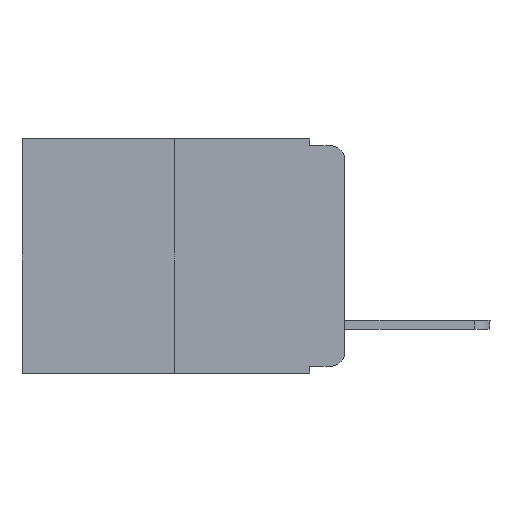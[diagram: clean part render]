
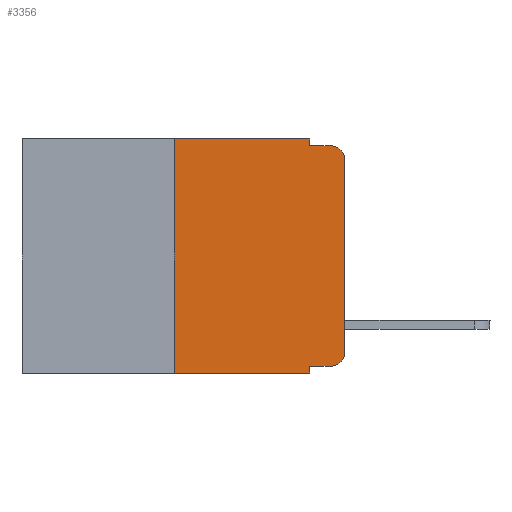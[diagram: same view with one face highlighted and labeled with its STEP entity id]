
A CAD part, left-side view. The second image highlights one B-rep face of the part: STEP entity #3356.
In plain terms, the highlighted planar face has unit normal (-1, 0, 0).
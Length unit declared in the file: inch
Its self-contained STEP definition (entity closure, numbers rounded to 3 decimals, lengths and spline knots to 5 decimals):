
#516 = CARTESIAN_POINT ( 'NONE',  ( 0., 0.051, 0. ) ) ;
#1097 = ORIENTED_EDGE ( 'NONE', *, *, #15260, .T. ) ;
#1399 = ORIENTED_EDGE ( 'NONE', *, *, #3674, .T. ) ;
#1534 = ORIENTED_EDGE ( 'NONE', *, *, #3552, .F. ) ;
#1713 = DIRECTION ( 'NONE',  ( -1., 0., 0. ) ) ;
#1716 = VERTEX_POINT ( 'NONE', #16718 ) ;
#1744 = LINE ( 'NONE', #8756, #10401 ) ;
#1872 = VECTOR ( 'NONE', #21773, 39.37008 ) ;
#2491 = PLANE ( 'NONE',  #20448 ) ;
#3356 = ADVANCED_FACE ( 'NONE', ( #13318 ), #2491, .F. ) ;
#3552 = EDGE_CURVE ( 'NONE', #8922, #5358, #19189, .T. ) ;
#3663 = DIRECTION ( 'NONE',  ( 0., 0., -1. ) ) ;
#3674 = EDGE_CURVE ( 'NONE', #6795, #16338, #4613, .T. ) ;
#3752 = CARTESIAN_POINT ( 'NONE',  ( 0., 0.473, -0.343 ) ) ;
#4172 = LINE ( 'NONE', #10744, #17664 ) ;
#4387 = DIRECTION ( 'NONE',  ( 0., 0., 1. ) ) ;
#4613 = LINE ( 'NONE', #11627, #20849 ) ;
#5263 = CARTESIAN_POINT ( 'NONE',  ( 0., 0.051, -0.333 ) ) ;
#5289 = CARTESIAN_POINT ( 'NONE',  ( 0., 0.02, -0.03 ) ) ;
#5358 = VERTEX_POINT ( 'NONE', #12371 ) ;
#5417 = CARTESIAN_POINT ( 'NONE',  ( 0., 0.25, -0.343 ) ) ;
#5496 = DIRECTION ( 'NONE',  ( 0., 0., -1. ) ) ;
#5788 = ORIENTED_EDGE ( 'NONE', *, *, #20070, .F. ) ;
#6242 = CARTESIAN_POINT ( 'NONE',  ( 0., 0.051, -0.01 ) ) ;
#6542 = VERTEX_POINT ( 'NONE', #11509 ) ;
#6795 = VERTEX_POINT ( 'NONE', #7782 ) ;
#7373 = ORIENTED_EDGE ( 'NONE', *, *, #12105, .T. ) ;
#7429 = DIRECTION ( 'NONE',  ( 0., -1., 0. ) ) ;
#7522 = DIRECTION ( 'NONE',  ( 0., 0., -1. ) ) ;
#7782 = CARTESIAN_POINT ( 'NONE',  ( 0., 0., -0.313 ) ) ;
#8155 = CIRCLE ( 'NONE', #21067, 0.02 ) ;
#8575 = ORIENTED_EDGE ( 'NONE', *, *, #13396, .F. ) ;
#8756 = CARTESIAN_POINT ( 'NONE',  ( 0., 0.473, 0. ) ) ;
#8760 = CARTESIAN_POINT ( 'NONE',  ( 0., 0.051, 0. ) ) ;
#8922 = VERTEX_POINT ( 'NONE', #6242 ) ;
#8944 = CARTESIAN_POINT ( 'NONE',  ( 0., 0.02, -0.313 ) ) ;
#8968 = VECTOR ( 'NONE', #5496, 39.37008 ) ;
#9504 = CARTESIAN_POINT ( 'NONE',  ( 0., 0.473, 0. ) ) ;
#9897 = CIRCLE ( 'NONE', #20600, 0.02 ) ;
#10401 = VECTOR ( 'NONE', #15806, 39.37008 ) ;
#10744 = CARTESIAN_POINT ( 'NONE',  ( 0., 0.051, 0. ) ) ;
#10857 = DIRECTION ( 'NONE',  ( 0., -1., 0. ) ) ;
#10921 = ORIENTED_EDGE ( 'NONE', *, *, #19192, .T. ) ;
#11509 = CARTESIAN_POINT ( 'NONE',  ( 0., 0.051, -0.333 ) ) ;
#11609 = CARTESIAN_POINT ( 'NONE',  ( 0., 0.25, 0. ) ) ;
#11627 = CARTESIAN_POINT ( 'NONE',  ( 0., 0., 0. ) ) ;
#11694 = VERTEX_POINT ( 'NONE', #5417 ) ;
#11960 = CARTESIAN_POINT ( 'NONE',  ( 0., 0.02, -0.333 ) ) ;
#12104 = CARTESIAN_POINT ( 'NONE',  ( 0., 0., -0.03 ) ) ;
#12105 = EDGE_CURVE ( 'NONE', #6542, #20189, #21035, .T. ) ;
#12227 = VECTOR ( 'NONE', #17567, 39.37008 ) ;
#12371 = CARTESIAN_POINT ( 'NONE',  ( 0., 0.02, -0.01 ) ) ;
#13111 = VECTOR ( 'NONE', #10857, 39.37008 ) ;
#13318 = FACE_OUTER_BOUND ( 'NONE', #18379, .T. ) ;
#13396 = EDGE_CURVE ( 'NONE', #6542, #19895, #21491, .T. ) ;
#14320 = ORIENTED_EDGE ( 'NONE', *, *, #17870, .F. ) ;
#14791 = ORIENTED_EDGE ( 'NONE', *, *, #17312, .F. ) ;
#15260 = EDGE_CURVE ( 'NONE', #16338, #5358, #9897, .T. ) ;
#15672 = EDGE_CURVE ( 'NONE', #11694, #19895, #19753, .T. ) ;
#15741 = CARTESIAN_POINT ( 'NONE',  ( 0., 0.051, -0.01 ) ) ;
#15806 = DIRECTION ( 'NONE',  ( 0., -1., 0. ) ) ;
#16290 = VERTEX_POINT ( 'NONE', #8760 ) ;
#16338 = VERTEX_POINT ( 'NONE', #12104 ) ;
#16550 = DIRECTION ( 'NONE',  ( 1., 0., 0. ) ) ;
#16718 = CARTESIAN_POINT ( 'NONE',  ( 0., 0.25, 0. ) ) ;
#17312 = EDGE_CURVE ( 'NONE', #16290, #8922, #4172, .T. ) ;
#17567 = DIRECTION ( 'NONE',  ( 0., -1., 0. ) ) ;
#17664 = VECTOR ( 'NONE', #7522, 39.37008 ) ;
#17870 = EDGE_CURVE ( 'NONE', #11694, #1716, #18407, .T. ) ;
#18224 = ORIENTED_EDGE ( 'NONE', *, *, #15672, .T. ) ;
#18379 = EDGE_LOOP ( 'NONE', ( #1399, #1097, #1534, #14791, #5788, #14320, #18224, #8575, #7373, #10921 ) ) ;
#18407 = LINE ( 'NONE', #11609, #1872 ) ;
#18538 = CARTESIAN_POINT ( 'NONE',  ( 0., 0.051, -0.343 ) ) ;
#18984 = DIRECTION ( 'NONE',  ( -1., 0., 0. ) ) ;
#19189 = LINE ( 'NONE', #15741, #13111 ) ;
#19192 = EDGE_CURVE ( 'NONE', #20189, #6795, #8155, .T. ) ;
#19753 = LINE ( 'NONE', #3752, #20785 ) ;
#19895 = VERTEX_POINT ( 'NONE', #18538 ) ;
#20070 = EDGE_CURVE ( 'NONE', #1716, #16290, #1744, .T. ) ;
#20189 = VERTEX_POINT ( 'NONE', #11960 ) ;
#20448 = AXIS2_PLACEMENT_3D ( 'NONE', #9504, #16550, #21847 ) ;
#20600 = AXIS2_PLACEMENT_3D ( 'NONE', #5289, #18984, #21176 ) ;
#20785 = VECTOR ( 'NONE', #7429, 39.37008 ) ;
#20849 = VECTOR ( 'NONE', #4387, 39.37008 ) ;
#21035 = LINE ( 'NONE', #5263, #12227 ) ;
#21067 = AXIS2_PLACEMENT_3D ( 'NONE', #8944, #1713, #3663 ) ;
#21176 = DIRECTION ( 'NONE',  ( 0., 0., -1. ) ) ;
#21491 = LINE ( 'NONE', #516, #8968 ) ;
#21773 = DIRECTION ( 'NONE',  ( 0., 0., 1. ) ) ;
#21847 = DIRECTION ( 'NONE',  ( 0., 0., -1. ) ) ;
